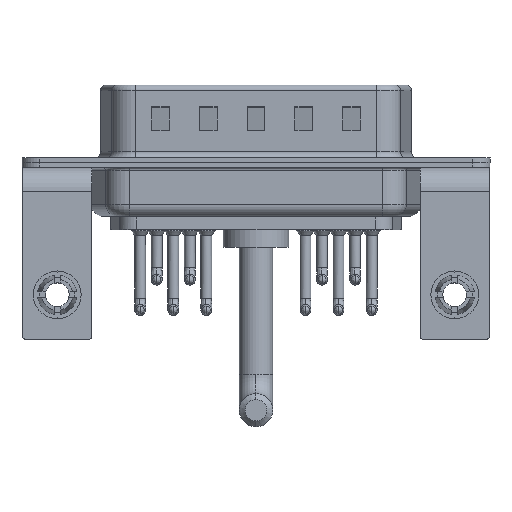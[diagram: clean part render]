
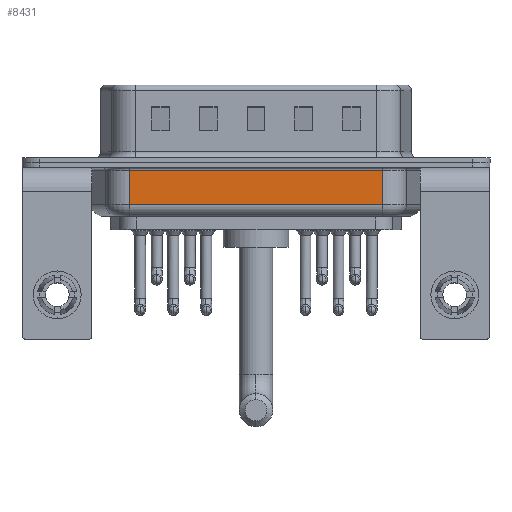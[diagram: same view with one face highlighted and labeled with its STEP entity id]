
A CAD part, front view. The second image highlights one B-rep face of the part: STEP entity #8431.
In plain terms, the highlighted planar face has unit normal (0, -1, 0).
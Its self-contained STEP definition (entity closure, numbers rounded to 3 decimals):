
#207 = DIRECTION ( 'NONE',  ( 0., 0., 1. ) ) ;
#334 = CARTESIAN_POINT ( 'NONE',  ( 6.031, -5.35, -4.5 ) ) ;
#776 = CARTESIAN_POINT ( 'NONE',  ( 27.269, -5.35, -4.5 ) ) ;
#1936 = ORIENTED_EDGE ( 'NONE', *, *, #23251, .T. ) ;
#2337 = VERTEX_POINT ( 'NONE', #11174 ) ;
#2959 = ORIENTED_EDGE ( 'NONE', *, *, #8555, .F. ) ;
#3026 = LINE ( 'NONE', #776, #18440 ) ;
#3691 = VECTOR ( 'NONE', #207, 1000. ) ;
#4417 = CARTESIAN_POINT ( 'NONE',  ( 6.031, -5.35, -3.5 ) ) ;
#7095 = LINE ( 'NONE', #14782, #19146 ) ;
#8247 = LINE ( 'NONE', #12027, #3691 ) ;
#8431 = ADVANCED_FACE ( 'NONE', ( #11901 ), #11667, .F. ) ;
#8451 = DIRECTION ( 'NONE',  ( 0., 0., 1. ) ) ;
#8555 = EDGE_CURVE ( 'NONE', #14282, #2337, #8247, .T. ) ;
#8822 = CARTESIAN_POINT ( 'NONE',  ( 27.269, -5.35, -0.65 ) ) ;
#9724 = DIRECTION ( 'NONE',  ( 1., 0., 0. ) ) ;
#11174 = CARTESIAN_POINT ( 'NONE',  ( 6.031, -5.35, -0.65 ) ) ;
#11667 = PLANE ( 'NONE',  #21399 ) ;
#11749 = VECTOR ( 'NONE', #9724, 1000. ) ;
#11901 = FACE_OUTER_BOUND ( 'NONE', #21895, .T. ) ;
#12027 = CARTESIAN_POINT ( 'NONE',  ( 6.031, -5.35, -4.5 ) ) ;
#12151 = DIRECTION ( 'NONE',  ( 0., 0., 1. ) ) ;
#12160 = ORIENTED_EDGE ( 'NONE', *, *, #18882, .T. ) ;
#13140 = EDGE_CURVE ( 'NONE', #16550, #21708, #3026, .T. ) ;
#13875 = CARTESIAN_POINT ( 'NONE',  ( 6.031, -5.35, -3.5 ) ) ;
#14282 = VERTEX_POINT ( 'NONE', #4417 ) ;
#14782 = CARTESIAN_POINT ( 'NONE',  ( 6.031, -5.35, -0.65 ) ) ;
#15411 = LINE ( 'NONE', #13875, #11749 ) ;
#16550 = VERTEX_POINT ( 'NONE', #17505 ) ;
#17505 = CARTESIAN_POINT ( 'NONE',  ( 27.269, -5.35, -3.5 ) ) ;
#18440 = VECTOR ( 'NONE', #8451, 1000. ) ;
#18882 = EDGE_CURVE ( 'NONE', #14282, #16550, #15411, .T. ) ;
#19146 = VECTOR ( 'NONE', #22249, 1000. ) ;
#21399 = AXIS2_PLACEMENT_3D ( 'NONE', #334, #23411, #12151 ) ;
#21708 = VERTEX_POINT ( 'NONE', #8822 ) ;
#21895 = EDGE_LOOP ( 'NONE', ( #2959, #12160, #23313, #1936 ) ) ;
#22249 = DIRECTION ( 'NONE',  ( -1., 0., 0. ) ) ;
#23251 = EDGE_CURVE ( 'NONE', #21708, #2337, #7095, .T. ) ;
#23313 = ORIENTED_EDGE ( 'NONE', *, *, #13140, .T. ) ;
#23411 = DIRECTION ( 'NONE',  ( 0., 1., 0. ) ) ;
